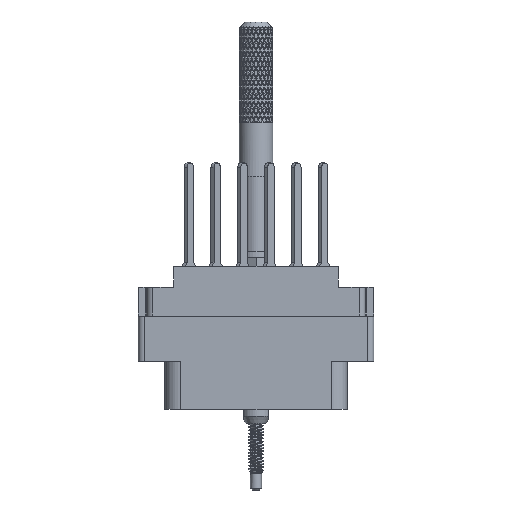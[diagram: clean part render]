
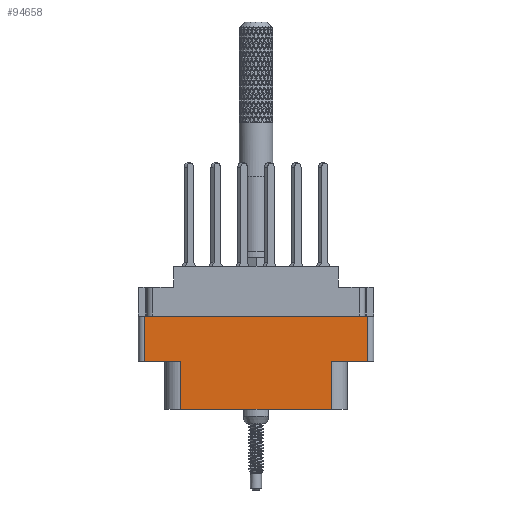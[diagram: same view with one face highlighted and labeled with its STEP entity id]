
A CAD part, front view. The second image highlights one B-rep face of the part: STEP entity #94658.
In plain terms, the highlighted planar face has unit normal (0, -1, 0).
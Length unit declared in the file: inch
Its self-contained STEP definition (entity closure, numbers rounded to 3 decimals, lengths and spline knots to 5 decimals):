
#172 = VERTEX_POINT ( 'NONE', #151964 ) ;
#4401 = ORIENTED_EDGE ( 'NONE', *, *, #67263, .T. ) ;
#6030 = LINE ( 'NONE', #35099, #25898 ) ;
#6360 = LINE ( 'NONE', #29819, #59435 ) ;
#7486 = ORIENTED_EDGE ( 'NONE', *, *, #47573, .F. ) ;
#7837 = VERTEX_POINT ( 'NONE', #97834 ) ;
#10338 = DIRECTION ( 'NONE',  ( 1., 0., 0. ) ) ;
#17897 = EDGE_CURVE ( 'NONE', #7837, #98913, #117687, .T. ) ;
#20177 = LINE ( 'NONE', #116399, #148736 ) ;
#21513 = CARTESIAN_POINT ( 'NONE',  ( -0.624, -0.343, -0.798 ) ) ;
#23042 = VECTOR ( 'NONE', #10338, 39.37008 ) ;
#24625 = DIRECTION ( 'NONE',  ( 0., 0., -1. ) ) ;
#25898 = VECTOR ( 'NONE', #163358, 39.37008 ) ;
#28604 = ORIENTED_EDGE ( 'NONE', *, *, #169398, .F. ) ;
#29819 = CARTESIAN_POINT ( 'NONE',  ( -0.656, -0.343, -0.277 ) ) ;
#30782 = VERTEX_POINT ( 'NONE', #115576 ) ;
#32534 = VERTEX_POINT ( 'NONE', #123706 ) ;
#33903 = ORIENTED_EDGE ( 'NONE', *, *, #145328, .T. ) ;
#35099 = CARTESIAN_POINT ( 'NONE',  ( 0., -0.343, -0.529 ) ) ;
#37207 = DIRECTION ( 'NONE',  ( 0., 0., -1. ) ) ;
#39249 = DIRECTION ( 'NONE',  ( 0., 0., -1. ) ) ;
#43038 = EDGE_CURVE ( 'NONE', #68179, #98913, #162792, .T. ) ;
#47573 = EDGE_CURVE ( 'NONE', #32534, #154147, #20177, .T. ) ;
#50699 = CARTESIAN_POINT ( 'NONE',  ( -0.42, -0.343, -0.798 ) ) ;
#51949 = CARTESIAN_POINT ( 'NONE',  ( 0.42, -0.343, -0.529 ) ) ;
#53522 = CARTESIAN_POINT ( 'NONE',  ( -0.42, -0.343, -0.529 ) ) ;
#54294 = EDGE_CURVE ( 'NONE', #154147, #172, #6360, .T. ) ;
#59435 = VECTOR ( 'NONE', #128908, 39.37008 ) ;
#67263 = EDGE_CURVE ( 'NONE', #88095, #68179, #118501, .T. ) ;
#68179 = VERTEX_POINT ( 'NONE', #50699 ) ;
#73136 = LINE ( 'NONE', #85958, #137446 ) ;
#74127 = VECTOR ( 'NONE', #39249, 39.37008 ) ;
#82070 = VECTOR ( 'NONE', #123669, 39.37008 ) ;
#85958 = CARTESIAN_POINT ( 'NONE',  ( 0.624, -0.343, -0.798 ) ) ;
#88095 = VERTEX_POINT ( 'NONE', #132543 ) ;
#90089 = ORIENTED_EDGE ( 'NONE', *, *, #54294, .F. ) ;
#94658 = ADVANCED_FACE ( 'NONE', ( #139788 ), #123300, .T. ) ;
#95199 = EDGE_CURVE ( 'NONE', #30782, #172, #73136, .T. ) ;
#97834 = CARTESIAN_POINT ( 'NONE',  ( 0.42, -0.343, -0.529 ) ) ;
#98913 = VERTEX_POINT ( 'NONE', #145732 ) ;
#104090 = ORIENTED_EDGE ( 'NONE', *, *, #17897, .F. ) ;
#107261 = DIRECTION ( 'NONE',  ( 0., -1., 0. ) ) ;
#115576 = CARTESIAN_POINT ( 'NONE',  ( 0.624, -0.343, -0.529 ) ) ;
#116399 = CARTESIAN_POINT ( 'NONE',  ( -0.624, -0.343, -0.798 ) ) ;
#117687 = LINE ( 'NONE', #51949, #168746 ) ;
#118501 = LINE ( 'NONE', #53522, #74127 ) ;
#118789 = CARTESIAN_POINT ( 'NONE',  ( 0., -0.343, -0.529 ) ) ;
#123300 = PLANE ( 'NONE',  #172493 ) ;
#123669 = DIRECTION ( 'NONE',  ( 1., 0., 0. ) ) ;
#123706 = CARTESIAN_POINT ( 'NONE',  ( -0.624, -0.343, -0.529 ) ) ;
#125136 = ORIENTED_EDGE ( 'NONE', *, *, #43038, .T. ) ;
#128908 = DIRECTION ( 'NONE',  ( 1., 0., 0. ) ) ;
#132543 = CARTESIAN_POINT ( 'NONE',  ( -0.42, -0.343, -0.529 ) ) ;
#132969 = EDGE_LOOP ( 'NONE', ( #4401, #125136, #104090, #28604, #149261, #90089, #7486, #33903 ) ) ;
#137446 = VECTOR ( 'NONE', #157147, 39.37008 ) ;
#139788 = FACE_OUTER_BOUND ( 'NONE', #132969, .T. ) ;
#145328 = EDGE_CURVE ( 'NONE', #32534, #88095, #155293, .T. ) ;
#145732 = CARTESIAN_POINT ( 'NONE',  ( 0.42, -0.343, -0.798 ) ) ;
#148736 = VECTOR ( 'NONE', #174607, 39.37008 ) ;
#149261 = ORIENTED_EDGE ( 'NONE', *, *, #95199, .T. ) ;
#151964 = CARTESIAN_POINT ( 'NONE',  ( 0.624, -0.343, -0.277 ) ) ;
#154147 = VERTEX_POINT ( 'NONE', #180069 ) ;
#155293 = LINE ( 'NONE', #118789, #82070 ) ;
#157147 = DIRECTION ( 'NONE',  ( 0., 0., 1. ) ) ;
#162792 = LINE ( 'NONE', #21513, #23042 ) ;
#163358 = DIRECTION ( 'NONE',  ( -1., 0., 0. ) ) ;
#168746 = VECTOR ( 'NONE', #24625, 39.37008 ) ;
#169398 = EDGE_CURVE ( 'NONE', #30782, #7837, #6030, .T. ) ;
#172493 = AXIS2_PLACEMENT_3D ( 'NONE', #177910, #107261, #37207 ) ;
#174607 = DIRECTION ( 'NONE',  ( 0., 0., 1. ) ) ;
#177910 = CARTESIAN_POINT ( 'NONE',  ( -0.624, -0.343, -0.798 ) ) ;
#180069 = CARTESIAN_POINT ( 'NONE',  ( -0.624, -0.343, -0.277 ) ) ;
